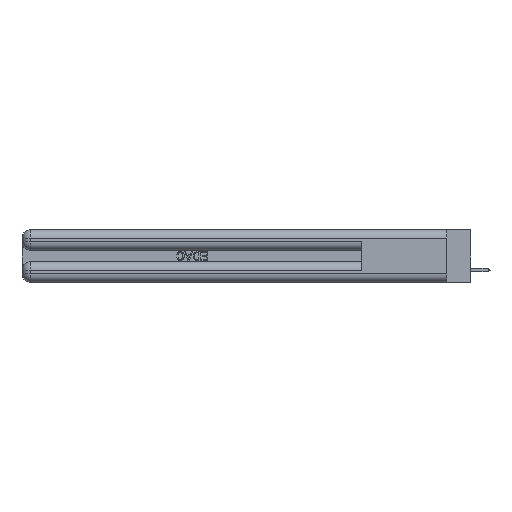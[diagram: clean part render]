
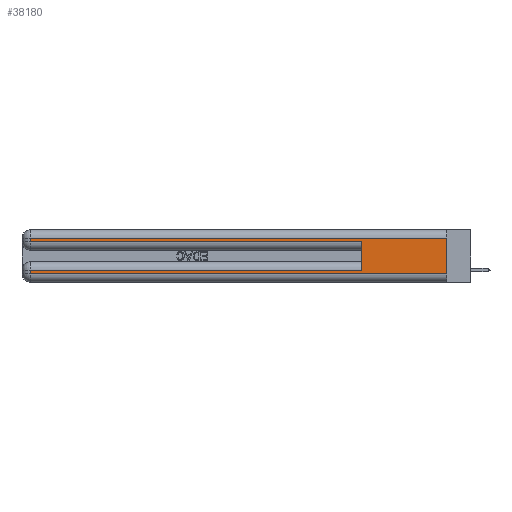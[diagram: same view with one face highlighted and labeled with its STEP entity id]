
A CAD part, left-side view. The second image highlights one B-rep face of the part: STEP entity #38180.
In plain terms, the highlighted planar face has unit normal (-1, 0, 0).
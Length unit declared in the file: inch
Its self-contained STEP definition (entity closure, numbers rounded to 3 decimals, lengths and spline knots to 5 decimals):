
#441 = CARTESIAN_POINT ( 'NONE',  ( 0., 0., 0.285 ) ) ;
#2266 = VECTOR ( 'NONE', #16451, 39.37008 ) ;
#3103 = PLANE ( 'NONE',  #14709 ) ;
#4130 = ORIENTED_EDGE ( 'NONE', *, *, #24726, .F. ) ;
#5118 = VERTEX_POINT ( 'NONE', #35790 ) ;
#5148 = CARTESIAN_POINT ( 'NONE',  ( 0., 0., 0.31 ) ) ;
#5182 = EDGE_CURVE ( 'NONE', #22975, #11038, #46972, .T. ) ;
#5263 = ORIENTED_EDGE ( 'NONE', *, *, #26480, .F. ) ;
#6334 = CARTESIAN_POINT ( 'NONE',  ( 0., 0.6, 0.285 ) ) ;
#6337 = LINE ( 'NONE', #19591, #14018 ) ;
#6741 = EDGE_LOOP ( 'NONE', ( #5263, #24995, #41423, #48144, #4130, #18868, #15228, #23174 ) ) ;
#8043 = LINE ( 'NONE', #41457, #45146 ) ;
#9145 = VERTEX_POINT ( 'NONE', #13403 ) ;
#11038 = VERTEX_POINT ( 'NONE', #21571 ) ;
#13017 = EDGE_CURVE ( 'NONE', #11038, #5118, #43591, .T. ) ;
#13403 = CARTESIAN_POINT ( 'NONE',  ( 0., 2.94, 0.06 ) ) ;
#14018 = VECTOR ( 'NONE', #41920, 39.37008 ) ;
#14709 = AXIS2_PLACEMENT_3D ( 'NONE', #29320, #29790, #25542 ) ;
#15228 = ORIENTED_EDGE ( 'NONE', *, *, #42160, .T. ) ;
#15283 = CARTESIAN_POINT ( 'NONE',  ( 0., 0., 0.37 ) ) ;
#16000 = CARTESIAN_POINT ( 'NONE',  ( 0., 0., 0.06 ) ) ;
#16267 = FACE_OUTER_BOUND ( 'NONE', #6741, .T. ) ;
#16290 = CARTESIAN_POINT ( 'NONE',  ( 0., 0.6, 0.145 ) ) ;
#16451 = DIRECTION ( 'NONE',  ( 0., 0., 1. ) ) ;
#16687 = DIRECTION ( 'NONE',  ( 0., 0., -1. ) ) ;
#18704 = VERTEX_POINT ( 'NONE', #37295 ) ;
#18868 = ORIENTED_EDGE ( 'NONE', *, *, #47612, .T. ) ;
#18955 = DIRECTION ( 'NONE',  ( 0., 1., 0. ) ) ;
#19554 = DIRECTION ( 'NONE',  ( 0., -1., 0. ) ) ;
#19591 = CARTESIAN_POINT ( 'NONE',  ( 0., 0., 0.06 ) ) ;
#21571 = CARTESIAN_POINT ( 'NONE',  ( 0., 2.94, 0.31 ) ) ;
#21990 = VECTOR ( 'NONE', #19554, 39.37008 ) ;
#22975 = VERTEX_POINT ( 'NONE', #25115 ) ;
#23174 = ORIENTED_EDGE ( 'NONE', *, *, #37053, .T. ) ;
#24153 = LINE ( 'NONE', #16290, #2266 ) ;
#24241 = VERTEX_POINT ( 'NONE', #6334 ) ;
#24726 = EDGE_CURVE ( 'NONE', #18704, #24241, #24153, .T. ) ;
#24995 = ORIENTED_EDGE ( 'NONE', *, *, #5182, .T. ) ;
#25115 = CARTESIAN_POINT ( 'NONE',  ( 0., 0., 0.31 ) ) ;
#25542 = DIRECTION ( 'NONE',  ( 0., 0., -1. ) ) ;
#26480 = EDGE_CURVE ( 'NONE', #22975, #40270, #33344, .T. ) ;
#27766 = DIRECTION ( 'NONE',  ( 0., 1., 0. ) ) ;
#28001 = DIRECTION ( 'NONE',  ( 0., 0., -1. ) ) ;
#28282 = EDGE_CURVE ( 'NONE', #5118, #24241, #46001, .T. ) ;
#28307 = LINE ( 'NONE', #39231, #34704 ) ;
#29320 = CARTESIAN_POINT ( 'NONE',  ( 0., 0., 0.37 ) ) ;
#29790 = DIRECTION ( 'NONE',  ( 1., 0., 0. ) ) ;
#33344 = LINE ( 'NONE', #15283, #41520 ) ;
#33608 = VERTEX_POINT ( 'NONE', #33829 ) ;
#33829 = CARTESIAN_POINT ( 'NONE',  ( 0., 2.94, 0.085 ) ) ;
#34704 = VECTOR ( 'NONE', #16687, 39.37008 ) ;
#35790 = CARTESIAN_POINT ( 'NONE',  ( 0., 2.94, 0.285 ) ) ;
#37053 = EDGE_CURVE ( 'NONE', #9145, #40270, #6337, .T. ) ;
#37295 = CARTESIAN_POINT ( 'NONE',  ( 0., 0.6, 0.085 ) ) ;
#37649 = CARTESIAN_POINT ( 'NONE',  ( 0., 2.94, 0.37 ) ) ;
#38180 = ADVANCED_FACE ( 'NONE', ( #16267 ), #3103, .F. ) ;
#39231 = CARTESIAN_POINT ( 'NONE',  ( 0., 2.94, 0.37 ) ) ;
#40270 = VERTEX_POINT ( 'NONE', #16000 ) ;
#41409 = DIRECTION ( 'NONE',  ( 0., 0., -1. ) ) ;
#41423 = ORIENTED_EDGE ( 'NONE', *, *, #13017, .T. ) ;
#41457 = CARTESIAN_POINT ( 'NONE',  ( 0., 0., 0.085 ) ) ;
#41520 = VECTOR ( 'NONE', #28001, 39.37008 ) ;
#41920 = DIRECTION ( 'NONE',  ( 0., -1., 0. ) ) ;
#42160 = EDGE_CURVE ( 'NONE', #33608, #9145, #28307, .T. ) ;
#42845 = VECTOR ( 'NONE', #27766, 39.37008 ) ;
#43591 = LINE ( 'NONE', #37649, #44139 ) ;
#44139 = VECTOR ( 'NONE', #41409, 39.37008 ) ;
#45146 = VECTOR ( 'NONE', #18955, 39.37008 ) ;
#46001 = LINE ( 'NONE', #441, #21990 ) ;
#46972 = LINE ( 'NONE', #5148, #42845 ) ;
#47612 = EDGE_CURVE ( 'NONE', #18704, #33608, #8043, .T. ) ;
#48144 = ORIENTED_EDGE ( 'NONE', *, *, #28282, .T. ) ;
